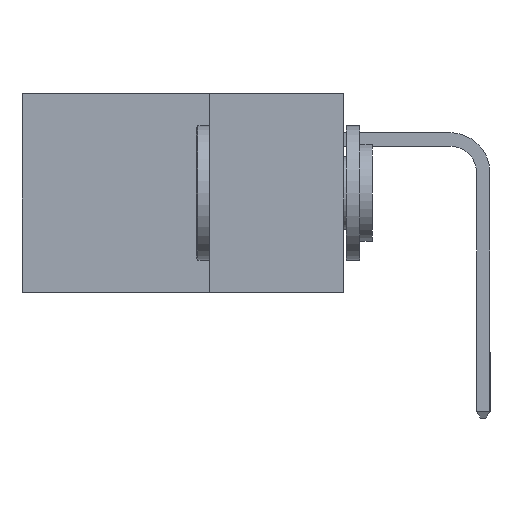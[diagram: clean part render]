
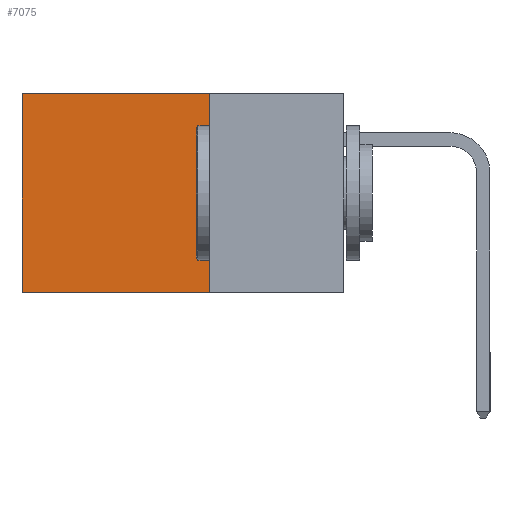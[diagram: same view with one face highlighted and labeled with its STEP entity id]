
A CAD part, left-side view. The second image highlights one B-rep face of the part: STEP entity #7075.
In plain terms, the highlighted planar face has unit normal (-1, 0, 0).
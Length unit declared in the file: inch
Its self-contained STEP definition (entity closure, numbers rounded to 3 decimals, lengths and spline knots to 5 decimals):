
#1178 = CARTESIAN_POINT ( 'NONE',  ( 0.298, 0.25, -0.37 ) ) ;
#2191 = VECTOR ( 'NONE', #8003, 39.37008 ) ;
#4058 = VERTEX_POINT ( 'NONE', #9357 ) ;
#4672 = VERTEX_POINT ( 'NONE', #22604 ) ;
#6986 = ORIENTED_EDGE ( 'NONE', *, *, #10863, .F. ) ;
#7075 = ADVANCED_FACE ( 'NONE', ( #12099 ), #19067, .F. ) ;
#7149 = LINE ( 'NONE', #16820, #2191 ) ;
#7884 = CARTESIAN_POINT ( 'NONE',  ( 0.298, 0.25, 0. ) ) ;
#8003 = DIRECTION ( 'NONE',  ( 0., 0., -1. ) ) ;
#9357 = CARTESIAN_POINT ( 'NONE',  ( 0.298, 0.6, 0. ) ) ;
#9422 = LINE ( 'NONE', #22066, #23070 ) ;
#9587 = DIRECTION ( 'NONE',  ( 0., 1., 0. ) ) ;
#10144 = DIRECTION ( 'NONE',  ( 0., 0., -1. ) ) ;
#10172 = EDGE_CURVE ( 'NONE', #20792, #4672, #9422, .T. ) ;
#10256 = EDGE_CURVE ( 'NONE', #4058, #4672, #7149, .T. ) ;
#10863 = EDGE_CURVE ( 'NONE', #21368, #20792, #13858, .T. ) ;
#11504 = DIRECTION ( 'NONE',  ( 0., 1., 0. ) ) ;
#12099 = FACE_OUTER_BOUND ( 'NONE', #14708, .T. ) ;
#12769 = VECTOR ( 'NONE', #13302, 39.37008 ) ;
#13302 = DIRECTION ( 'NONE',  ( 0., 0., -1. ) ) ;
#13716 = AXIS2_PLACEMENT_3D ( 'NONE', #15456, #20849, #10144 ) ;
#13858 = LINE ( 'NONE', #7884, #12769 ) ;
#14708 = EDGE_LOOP ( 'NONE', ( #19652, #15806, #6986, #21389 ) ) ;
#15456 = CARTESIAN_POINT ( 'NONE',  ( 0.298, 0.25, 0. ) ) ;
#15806 = ORIENTED_EDGE ( 'NONE', *, *, #10172, .F. ) ;
#16820 = CARTESIAN_POINT ( 'NONE',  ( 0.298, 0.6, 0. ) ) ;
#19067 = PLANE ( 'NONE',  #13716 ) ;
#19149 = CARTESIAN_POINT ( 'NONE',  ( 0.298, 0.25, 0. ) ) ;
#19652 = ORIENTED_EDGE ( 'NONE', *, *, #10256, .T. ) ;
#19824 = LINE ( 'NONE', #20395, #23367 ) ;
#20395 = CARTESIAN_POINT ( 'NONE',  ( 0.298, 0.25, 0. ) ) ;
#20792 = VERTEX_POINT ( 'NONE', #1178 ) ;
#20849 = DIRECTION ( 'NONE',  ( 1., 0., 0. ) ) ;
#21368 = VERTEX_POINT ( 'NONE', #19149 ) ;
#21389 = ORIENTED_EDGE ( 'NONE', *, *, #22861, .T. ) ;
#22066 = CARTESIAN_POINT ( 'NONE',  ( 0.298, 0.25, -0.37 ) ) ;
#22604 = CARTESIAN_POINT ( 'NONE',  ( 0.298, 0.6, -0.37 ) ) ;
#22861 = EDGE_CURVE ( 'NONE', #21368, #4058, #19824, .T. ) ;
#23070 = VECTOR ( 'NONE', #9587, 39.37008 ) ;
#23367 = VECTOR ( 'NONE', #11504, 39.37008 ) ;
